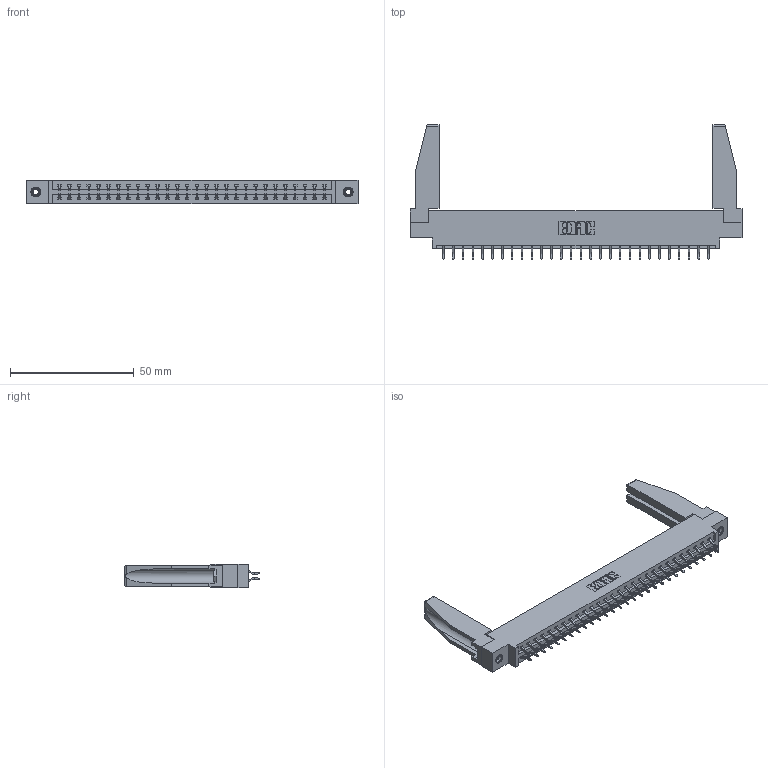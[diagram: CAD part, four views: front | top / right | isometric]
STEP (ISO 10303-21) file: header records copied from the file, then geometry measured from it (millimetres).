
FILE_DESCRIPTION (( 'STEP AP203' ), '1' );
FILE_NAME ('337-056-556-878.STEP', '2019-10-11T20:08:49', ( '' ), ( '' ), 'SwSTEP 2.0', 'SolidWorks 2016', '' );
FILE_SCHEMA (( 'CONFIG_CONTROL_DESIGN' ));
Length unit declared in the file: inch
Products named in the file (5): 345-292-001_556 Tail; 345-250-001_345-250-001-102; 307-220-078; 337 Part_0.170 Offset - 0.156 Dia-TI; 337-056-556-878
Assembly tree (61 placements, depth 2):
  337-056-556-878
    337 Part_0.170 Offset - 0.156 Dia-TI
    345-292-001_556 Tail  x56
    345-250-001_345-250-001-102  x2
    307-220-078  x2
Bounding box: 133.96 x 54.37 x 9.4 mm (x, y, z)
Volume: 17805 mm3; surface area: 19357.3 mm2
Topology: 61 solids, 61 shells, 3608 faces, 10677 edges, 7034 vertices
Faces by surface type: plane 2510, cylinder 1082, cone 12, torus 4
Entity records: 26312 total; most frequent: CARTESIAN_POINT 4460, ORIENTED_EDGE 4340, DIRECTION 3814, EDGE_CURVE 2170, LINE 1996, VECTOR 1996, VERTEX_POINT 1440, AXIS2_PLACEMENT_3D 909
